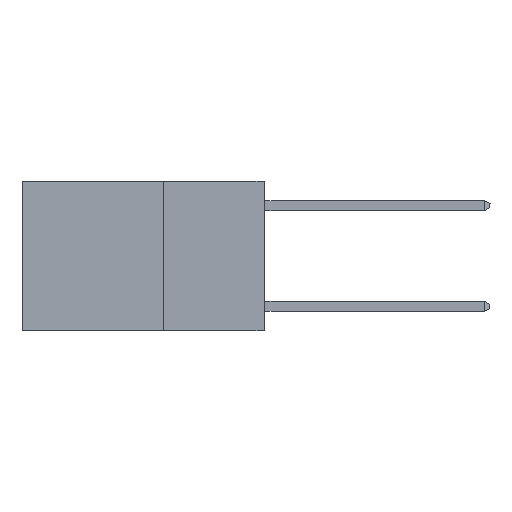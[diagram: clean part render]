
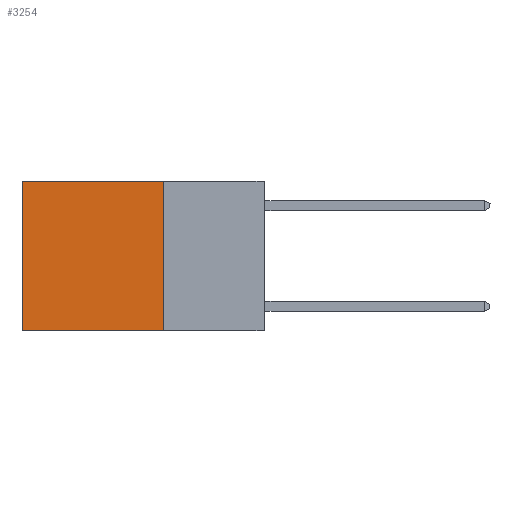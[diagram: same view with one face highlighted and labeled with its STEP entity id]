
A CAD part, left-side view. The second image highlights one B-rep face of the part: STEP entity #3254.
In plain terms, the highlighted planar face has unit normal (-1, 0, 0).
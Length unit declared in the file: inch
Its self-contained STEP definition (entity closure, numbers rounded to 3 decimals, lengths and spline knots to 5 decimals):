
#408 = VERTEX_POINT ( 'NONE', #1373 ) ;
#762 = CARTESIAN_POINT ( 'NONE',  ( 0.2625, 0.6, 0. ) ) ;
#1373 = CARTESIAN_POINT ( 'NONE',  ( 0.2625, 0.6, -0.37 ) ) ;
#1531 = VERTEX_POINT ( 'NONE', #762 ) ;
#1799 = VECTOR ( 'NONE', #25714, 39.37008 ) ;
#2292 = FACE_OUTER_BOUND ( 'NONE', #21951, .T. ) ;
#2441 = DIRECTION ( 'NONE',  ( 1., 0., 0. ) ) ;
#2999 = VERTEX_POINT ( 'NONE', #10821 ) ;
#3254 = ADVANCED_FACE ( 'NONE', ( #2292 ), #11721, .F. ) ;
#3486 = AXIS2_PLACEMENT_3D ( 'NONE', #21122, #2441, #11179 ) ;
#3696 = ORIENTED_EDGE ( 'NONE', *, *, #4534, .T. ) ;
#4534 = EDGE_CURVE ( 'NONE', #2999, #1531, #8991, .T. ) ;
#6907 = EDGE_CURVE ( 'NONE', #1531, #408, #26193, .T. ) ;
#8991 = LINE ( 'NONE', #18541, #21764 ) ;
#10821 = CARTESIAN_POINT ( 'NONE',  ( 0.2625, 0.25, 0. ) ) ;
#11179 = DIRECTION ( 'NONE',  ( 0., 0., -1. ) ) ;
#11400 = ORIENTED_EDGE ( 'NONE', *, *, #6907, .T. ) ;
#11721 = PLANE ( 'NONE',  #3486 ) ;
#11736 = EDGE_CURVE ( 'NONE', #27025, #408, #16007, .T. ) ;
#11918 = DIRECTION ( 'NONE',  ( 0., 1., 0. ) ) ;
#12417 = CARTESIAN_POINT ( 'NONE',  ( 0.2625, 0.25, 0. ) ) ;
#16007 = LINE ( 'NONE', #28152, #1799 ) ;
#17401 = ORIENTED_EDGE ( 'NONE', *, *, #11736, .F. ) ;
#17983 = CARTESIAN_POINT ( 'NONE',  ( 0.2625, 0.25, -0.37 ) ) ;
#18541 = CARTESIAN_POINT ( 'NONE',  ( 0.2625, 0.25, 0. ) ) ;
#21122 = CARTESIAN_POINT ( 'NONE',  ( 0.2625, 0.25, 0. ) ) ;
#21764 = VECTOR ( 'NONE', #11918, 39.37008 ) ;
#21878 = VECTOR ( 'NONE', #26451, 39.37008 ) ;
#21951 = EDGE_LOOP ( 'NONE', ( #11400, #17401, #25784, #3696 ) ) ;
#23451 = EDGE_CURVE ( 'NONE', #2999, #27025, #23832, .T. ) ;
#23575 = DIRECTION ( 'NONE',  ( 0., 0., -1. ) ) ;
#23832 = LINE ( 'NONE', #12417, #21878 ) ;
#25649 = VECTOR ( 'NONE', #23575, 39.37008 ) ;
#25714 = DIRECTION ( 'NONE',  ( 0., 1., 0. ) ) ;
#25784 = ORIENTED_EDGE ( 'NONE', *, *, #23451, .F. ) ;
#26193 = LINE ( 'NONE', #28626, #25649 ) ;
#26451 = DIRECTION ( 'NONE',  ( 0., 0., -1. ) ) ;
#27025 = VERTEX_POINT ( 'NONE', #17983 ) ;
#28152 = CARTESIAN_POINT ( 'NONE',  ( 0.2625, 0.25, -0.37 ) ) ;
#28626 = CARTESIAN_POINT ( 'NONE',  ( 0.2625, 0.6, 0. ) ) ;
